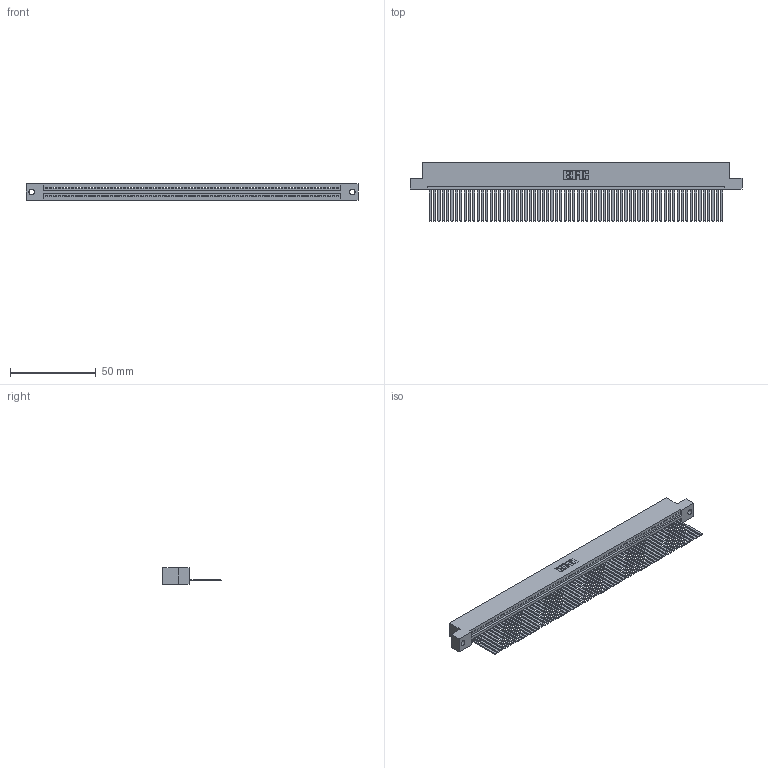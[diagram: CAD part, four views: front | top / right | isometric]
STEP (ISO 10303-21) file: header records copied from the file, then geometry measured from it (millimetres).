
FILE_DESCRIPTION (( 'STEP AP203' ), '1' );
FILE_NAME ('345-068-544-102.STEP', '2019-10-12T07:37:43', ( '' ), ( '' ), 'SwSTEP 2.0', 'SolidWorks 2016', '' );
FILE_SCHEMA (( 'CONFIG_CONTROL_DESIGN' ));
Length unit declared in the file: inch
Products named in the file (3): 345-068-544-102; 345-292-001_345-293-144; 345 Part_Flush Mounting Lugs - 0.128 Dia
Assembly tree (69 placements, depth 2):
  345-068-544-102
    345 Part_Flush Mounting Lugs - 0.128 Dia
    345-292-001_345-293-144  x68
Bounding box: 193.93 x 33.96 x 9.4 mm (x, y, z)
Volume: 19383.4 mm3; surface area: 28204.9 mm2
Topology: 69 solids, 69 shells, 3662 faces, 11085 edges, 7298 vertices
Faces by surface type: plane 2528, cylinder 1134
Entity records: 47497 total; most frequent: ORIENTED_EDGE 8234, CARTESIAN_POINT 8232, DIRECTION 7149, EDGE_CURVE 4117, VECTOR 3717, LINE 3717, VERTEX_POINT 2742, AXIS2_PLACEMENT_3D 1716
